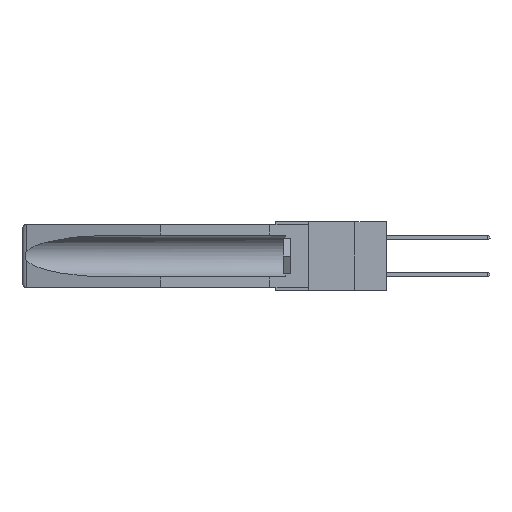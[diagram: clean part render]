
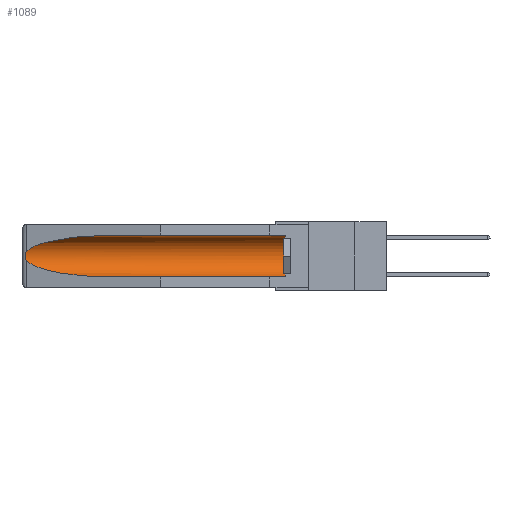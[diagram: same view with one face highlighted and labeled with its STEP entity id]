
A CAD part, left-side view. The second image highlights one B-rep face of the part: STEP entity #1089.
In plain terms, the highlighted cylindrical face has radius 2.857 mm (diameter 5.715 mm), a partial arc.
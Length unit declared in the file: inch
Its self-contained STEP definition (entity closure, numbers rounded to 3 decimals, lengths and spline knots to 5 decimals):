
#60 = EDGE_CURVE ( 'NONE', #13485, #13107, #5703, .T. ) ;
#103 = CARTESIAN_POINT ( 'NONE',  ( 0.25451, 1.48313, -0.09465 ) ) ;
#663 = CARTESIAN_POINT ( 'NONE',  ( 0.2673, 1.53269, -0.17917 ) ) ;
#953 = VECTOR ( 'NONE', #10377, 39.37008 ) ;
#1089 = ADVANCED_FACE ( 'NONE', ( #12386 ), #14361, .F. ) ;
#2081 = ORIENTED_EDGE ( 'NONE', *, *, #15963, .T. ) ;
#2266 = CARTESIAN_POINT ( 'NONE',  ( 0.2673, 1.5327, -0.16383 ) ) ;
#2683 = CARTESIAN_POINT ( 'NONE',  ( 0.26537, 1.52718, -0.14972 ) ) ;
#2882 = AXIS2_PLACEMENT_3D ( 'NONE', #12602, #7863, #15656 ) ;
#3175 = CARTESIAN_POINT ( 'NONE',  ( 0.26537, 1.52718, -0.14972 ) ) ;
#3379 = CARTESIAN_POINT ( 'NONE',  ( 0.155, 0.126, -0.284 ) ) ;
#3636 = ORIENTED_EDGE ( 'NONE', *, *, #60, .T. ) ;
#4220 = CIRCLE ( 'NONE', #2882, 0.1125 ) ;
#4231 = CARTESIAN_POINT ( 'NONE',  ( 0.155, -0.30754, -0.284 ) ) ;
#4692 = CARTESIAN_POINT ( 'NONE',  ( 0.155, 1.07973, -0.284 ) ) ;
#5084 = EDGE_LOOP ( 'NONE', ( #2081, #13348, #3636, #12629, #10031, #13794 ) ) ;
#5703 =( BOUNDED_CURVE ( )  B_SPLINE_CURVE ( 3, ( #6278, #15903, #14294, #17515 ),
 .UNSPECIFIED., .F., .T. ) 
 B_SPLINE_CURVE_WITH_KNOTS ( ( 4, 4 ),
 ( 0.1948, 1.5708 ),
 .UNSPECIFIED. ) 
 CURVE ( )  GEOMETRIC_REPRESENTATION_ITEM ( )  RATIONAL_B_SPLINE_CURVE ( ( 1., 0.848, 0.848, 1. ) ) 
 REPRESENTATION_ITEM ( '' )  );
#6194 = CARTESIAN_POINT ( 'NONE',  ( 0.21114, 1.30732, -0.059 ) ) ;
#6278 = CARTESIAN_POINT ( 'NONE',  ( 0.26537, 1.52718, -0.19328 ) ) ;
#7606 = CARTESIAN_POINT ( 'NONE',  ( 0.155, -0.30754, -0.1715 ) ) ;
#7863 = DIRECTION ( 'NONE',  ( 0., -1., 0. ) ) ;
#7968 = CARTESIAN_POINT ( 'NONE',  ( 0.155, 1.07973, -0.059 ) ) ;
#8242 = CARTESIAN_POINT ( 'NONE',  ( 0.155, 0.126, -0.059 ) ) ;
#8641 = CARTESIAN_POINT ( 'NONE',  ( 0.26537, 1.52718, -0.19328 ) ) ;
#8920 = DIRECTION ( 'NONE',  ( 0., 0., 1. ) ) ;
#10031 = ORIENTED_EDGE ( 'NONE', *, *, #10797, .T. ) ;
#10096 = CARTESIAN_POINT ( 'NONE',  ( 0.26655, 1.53094, -0.18657 ) ) ;
#10377 = DIRECTION ( 'NONE',  ( 0., 1., 0. ) ) ;
#10797 = EDGE_CURVE ( 'NONE', #13931, #16353, #4220, .T. ) ;
#11873 = EDGE_CURVE ( 'NONE', #13931, #13107, #12514, .T. ) ;
#12164 = EDGE_CURVE ( 'NONE', #16353, #12980, #17661, .T. ) ;
#12386 = FACE_OUTER_BOUND ( 'NONE', #5084, .T. ) ;
#12514 = LINE ( 'NONE', #4231, #16154 ) ;
#12602 = CARTESIAN_POINT ( 'NONE',  ( 0.155, 0.126, -0.1715 ) ) ;
#12629 = ORIENTED_EDGE ( 'NONE', *, *, #11873, .F. ) ;
#12980 = VERTEX_POINT ( 'NONE', #13712 ) ;
#13042 = VERTEX_POINT ( 'NONE', #2683 ) ;
#13107 = VERTEX_POINT ( 'NONE', #4692 ) ;
#13348 = ORIENTED_EDGE ( 'NONE', *, *, #16369, .T. ) ;
#13485 = VERTEX_POINT ( 'NONE', #17458 ) ;
#13712 = CARTESIAN_POINT ( 'NONE',  ( 0.155, 1.07973, -0.059 ) ) ;
#13794 = ORIENTED_EDGE ( 'NONE', *, *, #12164, .T. ) ;
#13931 = VERTEX_POINT ( 'NONE', #3379 ) ;
#14251 =( BOUNDED_CURVE ( )  B_SPLINE_CURVE ( 3, ( #7968, #6194, #103, #3175 ),
 .UNSPECIFIED., .F., .F. ) 
 B_SPLINE_CURVE_WITH_KNOTS ( ( 4, 4 ),
 ( 4.71239, 6.08839 ),
 .UNSPECIFIED. ) 
 CURVE ( )  GEOMETRIC_REPRESENTATION_ITEM ( )  RATIONAL_B_SPLINE_CURVE ( ( 1., 0.848, 0.848, 1. ) ) 
 REPRESENTATION_ITEM ( '' )  );
#14294 = CARTESIAN_POINT ( 'NONE',  ( 0.21114, 1.30732, -0.284 ) ) ;
#14361 = CYLINDRICAL_SURFACE ( 'NONE', #19920, 0.1125 ) ;
#14800 = CARTESIAN_POINT ( 'NONE',  ( 0.26597, 1.52961, -0.15275 ) ) ;
#15144 = DIRECTION ( 'NONE',  ( 0., 1., 0. ) ) ;
#15656 = DIRECTION ( 'NONE',  ( 0., 0., 1. ) ) ;
#15903 = CARTESIAN_POINT ( 'NONE',  ( 0.25451, 1.48313, -0.24835 ) ) ;
#15963 = EDGE_CURVE ( 'NONE', #12980, #13042, #14251, .T. ) ;
#16154 = VECTOR ( 'NONE', #18214, 39.37008 ) ;
#16280 = CARTESIAN_POINT ( 'NONE',  ( 0.26654, 1.53092, -0.15636 ) ) ;
#16353 = VERTEX_POINT ( 'NONE', #8242 ) ;
#16369 = EDGE_CURVE ( 'NONE', #13042, #13485, #19058, .T. ) ;
#16414 = CARTESIAN_POINT ( 'NONE',  ( 0.2675, 1.53308, -0.16763 ) ) ;
#16608 = CARTESIAN_POINT ( 'NONE',  ( 0.155, -0.30754, -0.059 ) ) ;
#17458 = CARTESIAN_POINT ( 'NONE',  ( 0.26537, 1.52718, -0.19328 ) ) ;
#17515 = CARTESIAN_POINT ( 'NONE',  ( 0.155, 1.07973, -0.284 ) ) ;
#17661 = LINE ( 'NONE', #16608, #953 ) ;
#18040 = CARTESIAN_POINT ( 'NONE',  ( 0.2675, 1.53308, -0.17534 ) ) ;
#18214 = DIRECTION ( 'NONE',  ( 0., 1., 0. ) ) ;
#19058 = B_SPLINE_CURVE_WITH_KNOTS ( 'NONE', 3,
 ( #19489, #14800, #16280, #2266, #16414, #18040, #663, #10096, #19560, #8641 ),
 .UNSPECIFIED., .F., .F.,
 ( 4, 2, 2, 2, 4 ),
 ( 0., 0.00029, 0.00058, 0.00087, 0.00117 ),
 .UNSPECIFIED. ) ;
#19489 = CARTESIAN_POINT ( 'NONE',  ( 0.26537, 1.52718, -0.14972 ) ) ;
#19560 = CARTESIAN_POINT ( 'NONE',  ( 0.26597, 1.5296, -0.19026 ) ) ;
#19920 = AXIS2_PLACEMENT_3D ( 'NONE', #7606, #15144, #8920 ) ;
